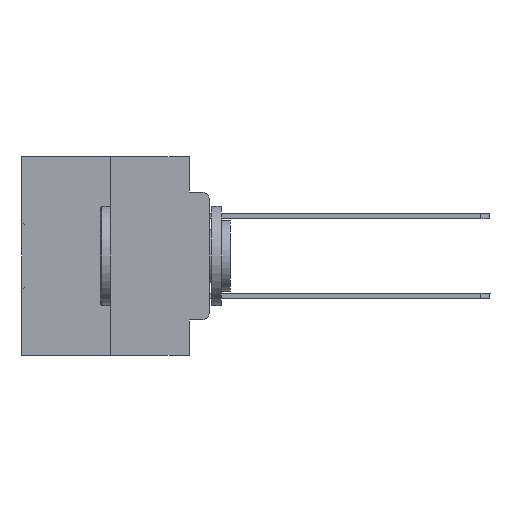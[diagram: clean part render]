
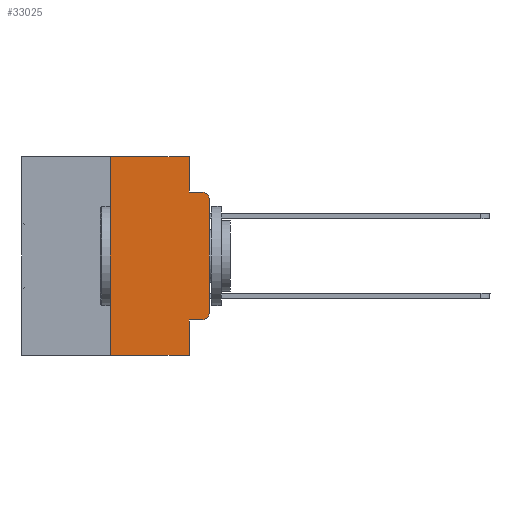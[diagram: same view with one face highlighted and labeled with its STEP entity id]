
A CAD part, left-side view. The second image highlights one B-rep face of the part: STEP entity #33025.
In plain terms, the highlighted planar face has unit normal (-1, 0, 0).
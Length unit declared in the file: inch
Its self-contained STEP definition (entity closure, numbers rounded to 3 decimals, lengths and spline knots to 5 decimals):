
#248 = CARTESIAN_POINT ( 'NONE',  ( 0., 0., -0.3915 ) ) ;
#1204 = CARTESIAN_POINT ( 'NONE',  ( 0., 0.473, 0. ) ) ;
#2099 = ORIENTED_EDGE ( 'NONE', *, *, #8949, .F. ) ;
#2554 = ORIENTED_EDGE ( 'NONE', *, *, #35338, .F. ) ;
#3338 = CARTESIAN_POINT ( 'NONE',  ( 0., 0.473, 0. ) ) ;
#3365 = LINE ( 'NONE', #25174, #19950 ) ;
#3615 = VERTEX_POINT ( 'NONE', #20462 ) ;
#5594 = LINE ( 'NONE', #27432, #32845 ) ;
#5673 = AXIS2_PLACEMENT_3D ( 'NONE', #21710, #29966, #26577 ) ;
#5837 = DIRECTION ( 'NONE',  ( 0., 0., -1. ) ) ;
#5868 = DIRECTION ( 'NONE',  ( 0., 0., -1. ) ) ;
#6047 = ORIENTED_EDGE ( 'NONE', *, *, #19913, .T. ) ;
#6548 = EDGE_CURVE ( 'NONE', #33341, #12293, #34376, .T. ) ;
#7991 = ORIENTED_EDGE ( 'NONE', *, *, #19907, .T. ) ;
#8053 = EDGE_CURVE ( 'NONE', #19228, #25655, #28391, .T. ) ;
#8371 = LINE ( 'NONE', #30561, #17228 ) ;
#8849 = ORIENTED_EDGE ( 'NONE', *, *, #6548, .T. ) ;
#8949 = EDGE_CURVE ( 'NONE', #16280, #29023, #3365, .T. ) ;
#9596 = EDGE_CURVE ( 'NONE', #3615, #12440, #17105, .T. ) ;
#9678 = CARTESIAN_POINT ( 'NONE',  ( 0., 0.25, 0. ) ) ;
#10105 = DIRECTION ( 'NONE',  ( 0., -1., 0. ) ) ;
#10654 = CARTESIAN_POINT ( 'NONE',  ( 0., 0.02, -0.4115 ) ) ;
#10871 = DIRECTION ( 'NONE',  ( 0., 0., -1. ) ) ;
#11654 = DIRECTION ( 'NONE',  ( 0., 0., 1. ) ) ;
#12293 = VERTEX_POINT ( 'NONE', #248 ) ;
#12440 = VERTEX_POINT ( 'NONE', #13610 ) ;
#12775 = CARTESIAN_POINT ( 'NONE',  ( 0., 0.051, -0.0885 ) ) ;
#13493 = VECTOR ( 'NONE', #11654, 39.37008 ) ;
#13610 = CARTESIAN_POINT ( 'NONE',  ( 0., 0.02, -0.0885 ) ) ;
#15302 = CARTESIAN_POINT ( 'NONE',  ( 0., 0.02, -0.3915 ) ) ;
#15326 = LINE ( 'NONE', #1204, #33882 ) ;
#16280 = VERTEX_POINT ( 'NONE', #34834 ) ;
#16517 = DIRECTION ( 'NONE',  ( 0., -1., 0. ) ) ;
#17105 = CIRCLE ( 'NONE', #5673, 0.02 ) ;
#17228 = VECTOR ( 'NONE', #22482, 39.37008 ) ;
#18965 = AXIS2_PLACEMENT_3D ( 'NONE', #15302, #19659, #10871 ) ;
#19228 = VERTEX_POINT ( 'NONE', #25613 ) ;
#19659 = DIRECTION ( 'NONE',  ( -1., 0., 0. ) ) ;
#19907 = EDGE_CURVE ( 'NONE', #12293, #3615, #32184, .T. ) ;
#19913 = EDGE_CURVE ( 'NONE', #26350, #29023, #8371, .T. ) ;
#19950 = VECTOR ( 'NONE', #5868, 39.37008 ) ;
#19991 = DIRECTION ( 'NONE',  ( 0., -1., 0. ) ) ;
#20462 = CARTESIAN_POINT ( 'NONE',  ( 0., 0., -0.1085 ) ) ;
#20623 = ORIENTED_EDGE ( 'NONE', *, *, #28270, .F. ) ;
#21046 = VECTOR ( 'NONE', #21529, 39.37008 ) ;
#21359 = EDGE_CURVE ( 'NONE', #33299, #19228, #15326, .T. ) ;
#21529 = DIRECTION ( 'NONE',  ( 0., 0., -1. ) ) ;
#21710 = CARTESIAN_POINT ( 'NONE',  ( 0., 0.02, -0.1085 ) ) ;
#21793 = VECTOR ( 'NONE', #35044, 39.37008 ) ;
#22468 = FACE_OUTER_BOUND ( 'NONE', #29487, .T. ) ;
#22482 = DIRECTION ( 'NONE',  ( 0., -1., 0. ) ) ;
#23048 = AXIS2_PLACEMENT_3D ( 'NONE', #3338, #25339, #5837 ) ;
#23170 = CARTESIAN_POINT ( 'NONE',  ( 0., 0.25, 0. ) ) ;
#23895 = CARTESIAN_POINT ( 'NONE',  ( 0., 0.051, -0.5 ) ) ;
#24115 = CARTESIAN_POINT ( 'NONE',  ( 0., 0., 0. ) ) ;
#24477 = CARTESIAN_POINT ( 'NONE',  ( 0., 0.25, -0.5 ) ) ;
#24922 = CARTESIAN_POINT ( 'NONE',  ( 0., 0.051, -0.0885 ) ) ;
#25174 = CARTESIAN_POINT ( 'NONE',  ( 0., 0.051, 0. ) ) ;
#25339 = DIRECTION ( 'NONE',  ( 1., 0., 0. ) ) ;
#25439 = VECTOR ( 'NONE', #10105, 39.37008 ) ;
#25613 = CARTESIAN_POINT ( 'NONE',  ( 0., 0.051, 0. ) ) ;
#25655 = VERTEX_POINT ( 'NONE', #24922 ) ;
#26350 = VERTEX_POINT ( 'NONE', #24477 ) ;
#26377 = LINE ( 'NONE', #12775, #25439 ) ;
#26577 = DIRECTION ( 'NONE',  ( 0., 0., -1. ) ) ;
#27309 = ORIENTED_EDGE ( 'NONE', *, *, #8053, .F. ) ;
#27432 = CARTESIAN_POINT ( 'NONE',  ( 0., 0.051, -0.4115 ) ) ;
#27491 = PLANE ( 'NONE',  #23048 ) ;
#27790 = ORIENTED_EDGE ( 'NONE', *, *, #9596, .T. ) ;
#28270 = EDGE_CURVE ( 'NONE', #25655, #12440, #26377, .T. ) ;
#28391 = LINE ( 'NONE', #33928, #21046 ) ;
#29023 = VERTEX_POINT ( 'NONE', #23895 ) ;
#29487 = EDGE_LOOP ( 'NONE', ( #7991, #27790, #20623, #27309, #33583, #2554, #6047, #2099, #30440, #8849 ) ) ;
#29695 = EDGE_CURVE ( 'NONE', #16280, #33341, #5594, .T. ) ;
#29966 = DIRECTION ( 'NONE',  ( -1., 0., 0. ) ) ;
#30440 = ORIENTED_EDGE ( 'NONE', *, *, #29695, .T. ) ;
#30561 = CARTESIAN_POINT ( 'NONE',  ( 0., 0.473, -0.5 ) ) ;
#32184 = LINE ( 'NONE', #24115, #21793 ) ;
#32786 = LINE ( 'NONE', #9678, #13493 ) ;
#32845 = VECTOR ( 'NONE', #16517, 39.37008 ) ;
#33025 = ADVANCED_FACE ( 'NONE', ( #22468 ), #27491, .F. ) ;
#33299 = VERTEX_POINT ( 'NONE', #23170 ) ;
#33341 = VERTEX_POINT ( 'NONE', #10654 ) ;
#33583 = ORIENTED_EDGE ( 'NONE', *, *, #21359, .F. ) ;
#33882 = VECTOR ( 'NONE', #19991, 39.37008 ) ;
#33928 = CARTESIAN_POINT ( 'NONE',  ( 0., 0.051, 0. ) ) ;
#34376 = CIRCLE ( 'NONE', #18965, 0.02 ) ;
#34834 = CARTESIAN_POINT ( 'NONE',  ( 0., 0.051, -0.4115 ) ) ;
#35044 = DIRECTION ( 'NONE',  ( 0., 0., 1. ) ) ;
#35338 = EDGE_CURVE ( 'NONE', #26350, #33299, #32786, .T. ) ;
